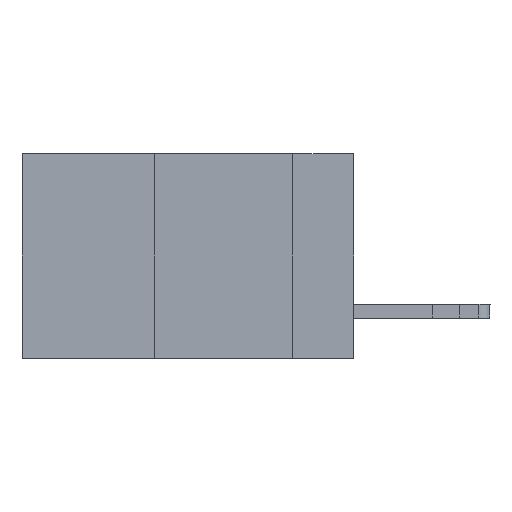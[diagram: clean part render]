
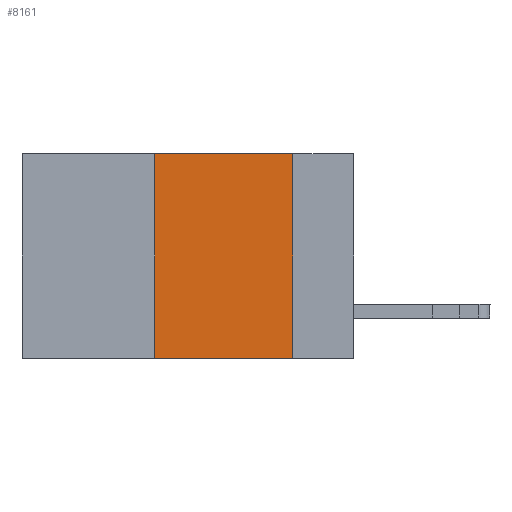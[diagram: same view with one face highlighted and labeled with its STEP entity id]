
A CAD part, left-side view. The second image highlights one B-rep face of the part: STEP entity #8161.
In plain terms, the highlighted planar face has unit normal (-1, 0, 0).
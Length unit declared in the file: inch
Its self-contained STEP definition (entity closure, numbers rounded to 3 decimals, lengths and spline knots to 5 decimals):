
#544 = EDGE_LOOP ( 'NONE', ( #1274, #12345, #11794, #3675 ) ) ;
#1274 = ORIENTED_EDGE ( 'NONE', *, *, #14982, .F. ) ;
#1806 = LINE ( 'NONE', #9058, #10687 ) ;
#3675 = ORIENTED_EDGE ( 'NONE', *, *, #4246, .T. ) ;
#3686 = VERTEX_POINT ( 'NONE', #4762 ) ;
#3722 = LINE ( 'NONE', #6012, #8186 ) ;
#4246 = EDGE_CURVE ( 'NONE', #16603, #3686, #14202, .T. ) ;
#4762 = CARTESIAN_POINT ( 'NONE',  ( 0., 0.11, -0.37 ) ) ;
#4823 = DIRECTION ( 'NONE',  ( 0., 0., -1. ) ) ;
#6012 = CARTESIAN_POINT ( 'NONE',  ( 0., 0.11, 0. ) ) ;
#6567 = CARTESIAN_POINT ( 'NONE',  ( 0., 0.36, 0. ) ) ;
#6908 = DIRECTION ( 'NONE',  ( 1., 0., 0. ) ) ;
#7110 = FACE_OUTER_BOUND ( 'NONE', #544, .T. ) ;
#7644 = AXIS2_PLACEMENT_3D ( 'NONE', #9586, #6908, #16273 ) ;
#7731 = VECTOR ( 'NONE', #9206, 39.37008 ) ;
#8161 = ADVANCED_FACE ( 'NONE', ( #7110 ), #14941, .F. ) ;
#8186 = VECTOR ( 'NONE', #4823, 39.37008 ) ;
#8274 = CARTESIAN_POINT ( 'NONE',  ( 0., 0.36, 0. ) ) ;
#8668 = VERTEX_POINT ( 'NONE', #9576 ) ;
#9058 = CARTESIAN_POINT ( 'NONE',  ( 0., 0.6, 0. ) ) ;
#9206 = DIRECTION ( 'NONE',  ( 0., 0., 1. ) ) ;
#9576 = CARTESIAN_POINT ( 'NONE',  ( 0., 0.11, 0. ) ) ;
#9586 = CARTESIAN_POINT ( 'NONE',  ( 0., 0.6, 0. ) ) ;
#9722 = EDGE_CURVE ( 'NONE', #14032, #8668, #1806, .T. ) ;
#9827 = EDGE_CURVE ( 'NONE', #16603, #14032, #10259, .T. ) ;
#10259 = LINE ( 'NONE', #6567, #7731 ) ;
#10632 = VECTOR ( 'NONE', #13338, 39.37008 ) ;
#10687 = VECTOR ( 'NONE', #14660, 39.37008 ) ;
#11794 = ORIENTED_EDGE ( 'NONE', *, *, #9827, .F. ) ;
#12345 = ORIENTED_EDGE ( 'NONE', *, *, #9722, .F. ) ;
#13338 = DIRECTION ( 'NONE',  ( 0., -1., 0. ) ) ;
#13493 = CARTESIAN_POINT ( 'NONE',  ( 0., 0.36, -0.37 ) ) ;
#14032 = VERTEX_POINT ( 'NONE', #8274 ) ;
#14202 = LINE ( 'NONE', #16167, #10632 ) ;
#14660 = DIRECTION ( 'NONE',  ( 0., -1., 0. ) ) ;
#14941 = PLANE ( 'NONE',  #7644 ) ;
#14982 = EDGE_CURVE ( 'NONE', #8668, #3686, #3722, .T. ) ;
#16167 = CARTESIAN_POINT ( 'NONE',  ( 0., 0.6, -0.37 ) ) ;
#16273 = DIRECTION ( 'NONE',  ( 0., 0., -1. ) ) ;
#16603 = VERTEX_POINT ( 'NONE', #13493 ) ;
